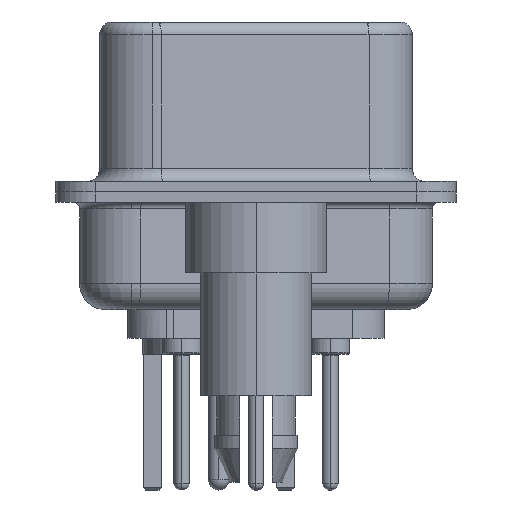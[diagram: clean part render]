
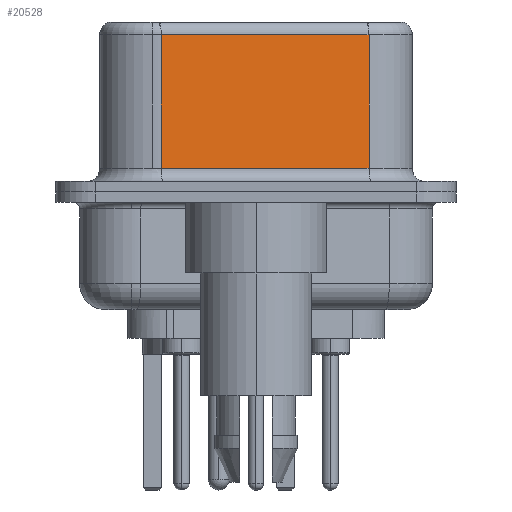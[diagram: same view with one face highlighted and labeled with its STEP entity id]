
A CAD part, left-side view. The second image highlights one B-rep face of the part: STEP entity #20528.
In plain terms, the highlighted planar face has unit normal (-0.985, -0.174, 0).
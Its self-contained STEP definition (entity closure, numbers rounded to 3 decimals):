
#1961 = CARTESIAN_POINT ( 'NONE',  ( 5.132, -4.322, 0.9 ) ) ;
#2262 = CARTESIAN_POINT ( 'NONE',  ( 5.132, -4.322, 6.52 ) ) ;
#3498 = VECTOR ( 'NONE', #13380, 1000. ) ;
#3573 = LINE ( 'NONE', #26907, #28866 ) ;
#3593 = VERTEX_POINT ( 'NONE', #1961 ) ;
#4763 = DIRECTION ( 'NONE',  ( 0., 0., -1. ) ) ;
#5488 = LINE ( 'NONE', #2262, #24269 ) ;
#6650 = EDGE_CURVE ( 'NONE', #8036, #12659, #27305, .T. ) ;
#7153 = EDGE_CURVE ( 'NONE', #12659, #19504, #16598, .T. ) ;
#8036 = VERTEX_POINT ( 'NONE', #30437 ) ;
#8579 = VECTOR ( 'NONE', #17592, 1000. ) ;
#8888 = CARTESIAN_POINT ( 'NONE',  ( 5.132, -4.322, 6.52 ) ) ;
#9448 = ORIENTED_EDGE ( 'NONE', *, *, #23251, .T. ) ;
#9840 = DIRECTION ( 'NONE',  ( 0.174, -0.985, 0. ) ) ;
#11389 = DIRECTION ( 'NONE',  ( -0.174, 0.985, 0. ) ) ;
#11551 = AXIS2_PLACEMENT_3D ( 'NONE', #8888, #26007, #11389 ) ;
#12659 = VERTEX_POINT ( 'NONE', #19567 ) ;
#13380 = DIRECTION ( 'NONE',  ( 0., 0., -1. ) ) ;
#13806 = CARTESIAN_POINT ( 'NONE',  ( 3.73, 3.628, 6.52 ) ) ;
#16598 = LINE ( 'NONE', #13806, #3498 ) ;
#17592 = DIRECTION ( 'NONE',  ( -0.174, 0.985, 0. ) ) ;
#19504 = VERTEX_POINT ( 'NONE', #21215 ) ;
#19567 = CARTESIAN_POINT ( 'NONE',  ( 3.73, 3.628, 6.02 ) ) ;
#20295 = ORIENTED_EDGE ( 'NONE', *, *, #28098, .F. ) ;
#20528 = ADVANCED_FACE ( 'NONE', ( #25553 ), #21121, .F. ) ;
#20929 = ORIENTED_EDGE ( 'NONE', *, *, #7153, .T. ) ;
#21121 = PLANE ( 'NONE',  #11551 ) ;
#21215 = CARTESIAN_POINT ( 'NONE',  ( 3.73, 3.628, 0.9 ) ) ;
#21517 = EDGE_LOOP ( 'NONE', ( #20295, #29714, #20929, #9448 ) ) ;
#23251 = EDGE_CURVE ( 'NONE', #19504, #3593, #3573, .T. ) ;
#24158 = CARTESIAN_POINT ( 'NONE',  ( 5.132, -4.322, 6.02 ) ) ;
#24269 = VECTOR ( 'NONE', #4763, 1000. ) ;
#25553 = FACE_OUTER_BOUND ( 'NONE', #21517, .T. ) ;
#26007 = DIRECTION ( 'NONE',  ( 0.985, 0.174, 0. ) ) ;
#26907 = CARTESIAN_POINT ( 'NONE',  ( 5.132, -4.322, 0.9 ) ) ;
#27305 = LINE ( 'NONE', #24158, #8579 ) ;
#28098 = EDGE_CURVE ( 'NONE', #8036, #3593, #5488, .T. ) ;
#28866 = VECTOR ( 'NONE', #9840, 1000. ) ;
#29714 = ORIENTED_EDGE ( 'NONE', *, *, #6650, .T. ) ;
#30437 = CARTESIAN_POINT ( 'NONE',  ( 5.132, -4.322, 6.02 ) ) ;
